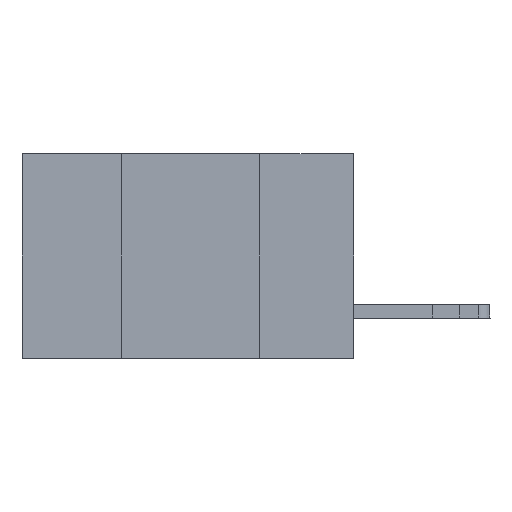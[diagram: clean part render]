
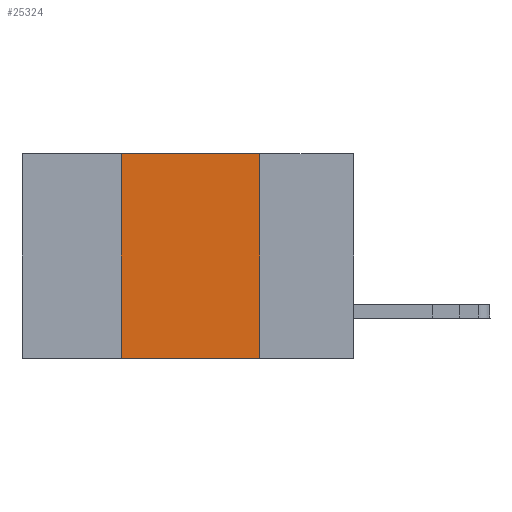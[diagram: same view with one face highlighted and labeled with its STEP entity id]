
A CAD part, left-side view. The second image highlights one B-rep face of the part: STEP entity #25324.
In plain terms, the highlighted planar face has unit normal (-1, 0, 0).
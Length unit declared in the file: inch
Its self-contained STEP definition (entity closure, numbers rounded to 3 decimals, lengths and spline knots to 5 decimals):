
#79 = EDGE_LOOP ( 'NONE', ( #1967, #14519, #33035, #33651 ) ) ;
#1371 = LINE ( 'NONE', #22086, #23581 ) ;
#1491 = VERTEX_POINT ( 'NONE', #15399 ) ;
#1967 = ORIENTED_EDGE ( 'NONE', *, *, #33953, .F. ) ;
#2581 = CARTESIAN_POINT ( 'NONE',  ( 0., 0.17, -0.37 ) ) ;
#2966 = DIRECTION ( 'NONE',  ( 0., -1., 0. ) ) ;
#3260 = DIRECTION ( 'NONE',  ( 0., 0., -1. ) ) ;
#3609 = VECTOR ( 'NONE', #2966, 39.37008 ) ;
#3772 = CARTESIAN_POINT ( 'NONE',  ( 0., 0.6, 0. ) ) ;
#7240 = VERTEX_POINT ( 'NONE', #26327 ) ;
#7242 = VECTOR ( 'NONE', #28251, 39.37008 ) ;
#11222 = PLANE ( 'NONE',  #30382 ) ;
#11563 = VERTEX_POINT ( 'NONE', #2581 ) ;
#11904 = FACE_OUTER_BOUND ( 'NONE', #79, .T. ) ;
#12550 = LINE ( 'NONE', #14787, #7242 ) ;
#14519 = ORIENTED_EDGE ( 'NONE', *, *, #26587, .F. ) ;
#14787 = CARTESIAN_POINT ( 'NONE',  ( 0., 0.17, 0. ) ) ;
#15399 = CARTESIAN_POINT ( 'NONE',  ( 0., 0.42, 0. ) ) ;
#17037 = VECTOR ( 'NONE', #33827, 39.37008 ) ;
#20533 = LINE ( 'NONE', #26042, #17037 ) ;
#20910 = CARTESIAN_POINT ( 'NONE',  ( 0., 0.6, -0.37 ) ) ;
#21273 = LINE ( 'NONE', #20910, #3609 ) ;
#22086 = CARTESIAN_POINT ( 'NONE',  ( 0., 0.6, 0. ) ) ;
#22433 = DIRECTION ( 'NONE',  ( 1., 0., 0. ) ) ;
#22800 = CARTESIAN_POINT ( 'NONE',  ( 0., 0.42, -0.37 ) ) ;
#23485 = EDGE_CURVE ( 'NONE', #33547, #11563, #21273, .T. ) ;
#23581 = VECTOR ( 'NONE', #25183, 39.37008 ) ;
#25183 = DIRECTION ( 'NONE',  ( 0., -1., 0. ) ) ;
#25324 = ADVANCED_FACE ( 'NONE', ( #11904 ), #11222, .F. ) ;
#26042 = CARTESIAN_POINT ( 'NONE',  ( 0., 0.42, 0. ) ) ;
#26327 = CARTESIAN_POINT ( 'NONE',  ( 0., 0.17, 0. ) ) ;
#26587 = EDGE_CURVE ( 'NONE', #1491, #7240, #1371, .T. ) ;
#28251 = DIRECTION ( 'NONE',  ( 0., 0., -1. ) ) ;
#30382 = AXIS2_PLACEMENT_3D ( 'NONE', #3772, #22433, #3260 ) ;
#33035 = ORIENTED_EDGE ( 'NONE', *, *, #33583, .F. ) ;
#33547 = VERTEX_POINT ( 'NONE', #22800 ) ;
#33583 = EDGE_CURVE ( 'NONE', #33547, #1491, #20533, .T. ) ;
#33651 = ORIENTED_EDGE ( 'NONE', *, *, #23485, .T. ) ;
#33827 = DIRECTION ( 'NONE',  ( 0., 0., 1. ) ) ;
#33953 = EDGE_CURVE ( 'NONE', #7240, #11563, #12550, .T. ) ;
